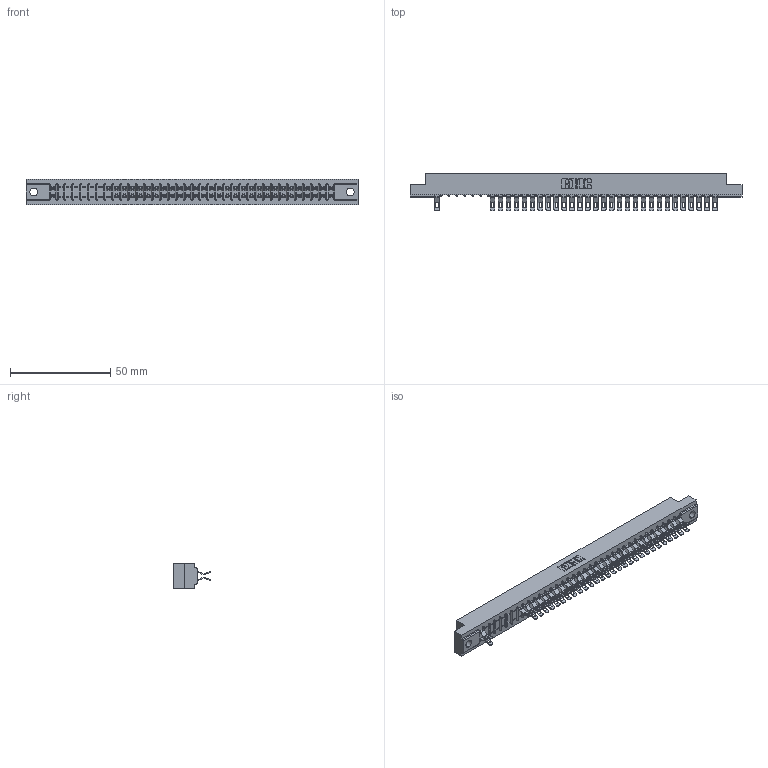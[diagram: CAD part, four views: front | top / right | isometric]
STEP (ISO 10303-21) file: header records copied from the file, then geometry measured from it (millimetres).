
FILE_DESCRIPTION (( 'STEP AP203' ), '1' );
FILE_NAME ('307-072-555-204.STEP', '2018-08-06T15:35:33', ( '' ), ( '' ), 'SwSTEP 2.0', 'SolidWorks 2016', '' );
FILE_SCHEMA (( 'CONFIG_CONTROL_DESIGN' ));
Length unit declared in the file: inch
Products named in the file (3): 307-290-001_555; 307-072-555-204; 307 Part_.156 Dia Mounting Holes
Assembly tree (60 placements, depth 2):
  307-072-555-204
    307 Part_.156 Dia Mounting Holes
    307-290-001_555  x59
Bounding box: 165.66 x 18.75 x 12.7 mm (x, y, z)
Volume: 17474.9 mm3; surface area: 20964.2 mm2
Topology: 60 solids, 60 shells, 3898 faces, 11454 edges, 7456 vertices
Faces by surface type: plane 2168, cylinder 1656, sphere 74
Entity records: 33293 total; most frequent: CARTESIAN_POINT 5513, ORIENTED_EDGE 5476, DIRECTION 5388, EDGE_CURVE 2738, VECTOR 2094, LINE 2094, VERTEX_POINT 1772, AXIS2_PLACEMENT_3D 1647
